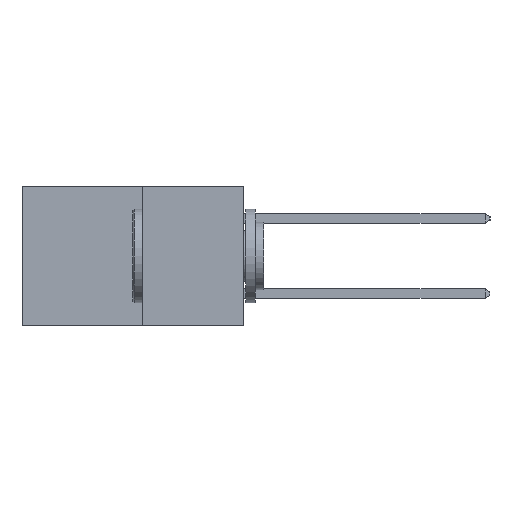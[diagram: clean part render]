
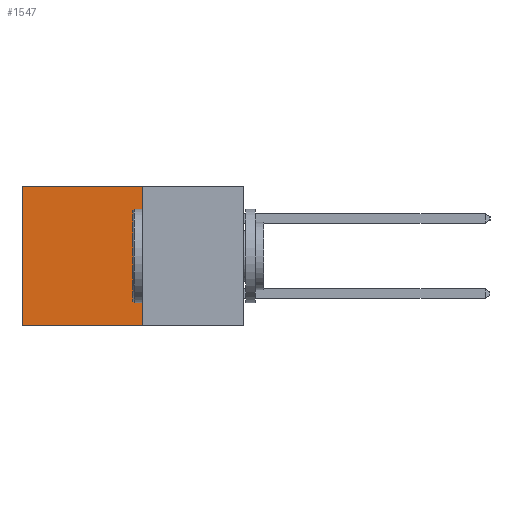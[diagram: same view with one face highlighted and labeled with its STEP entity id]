
A CAD part, left-side view. The second image highlights one B-rep face of the part: STEP entity #1547.
In plain terms, the highlighted planar face has unit normal (-1, 0, 0).
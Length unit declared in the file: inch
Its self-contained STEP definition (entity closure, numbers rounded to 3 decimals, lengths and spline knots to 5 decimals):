
#429 = DIRECTION ( 'NONE',  ( 0., 1., 0. ) ) ;
#512 = LINE ( 'NONE', #8108, #9013 ) ;
#549 = CARTESIAN_POINT ( 'NONE',  ( 0.277, 0.27, -0.37 ) ) ;
#713 = ORIENTED_EDGE ( 'NONE', *, *, #4746, .F. ) ;
#1438 = EDGE_LOOP ( 'NONE', ( #6403, #713, #5335, #3864 ) ) ;
#1547 = ADVANCED_FACE ( 'NONE', ( #10378 ), #9624, .F. ) ;
#2366 = VERTEX_POINT ( 'NONE', #4047 ) ;
#3277 = CARTESIAN_POINT ( 'NONE',  ( 0.277, 0.27, -0.37 ) ) ;
#3645 = VECTOR ( 'NONE', #9243, 39.37008 ) ;
#3669 = EDGE_CURVE ( 'NONE', #6600, #9854, #10210, .T. ) ;
#3829 = DIRECTION ( 'NONE',  ( 0., 0., -1. ) ) ;
#3864 = ORIENTED_EDGE ( 'NONE', *, *, #3669, .T. ) ;
#3939 = CARTESIAN_POINT ( 'NONE',  ( 0.277, 0.59, -0.37 ) ) ;
#4047 = CARTESIAN_POINT ( 'NONE',  ( 0.277, 0.59, -0.37 ) ) ;
#4356 = EDGE_CURVE ( 'NONE', #9854, #2366, #10320, .T. ) ;
#4531 = VECTOR ( 'NONE', #429, 39.37008 ) ;
#4746 = EDGE_CURVE ( 'NONE', #5985, #2366, #8927, .T. ) ;
#5112 = CARTESIAN_POINT ( 'NONE',  ( 0.277, 0.59, 0. ) ) ;
#5335 = ORIENTED_EDGE ( 'NONE', *, *, #10617, .F. ) ;
#5985 = VERTEX_POINT ( 'NONE', #7421 ) ;
#6403 = ORIENTED_EDGE ( 'NONE', *, *, #4356, .T. ) ;
#6469 = DIRECTION ( 'NONE',  ( 0., 0., -1. ) ) ;
#6600 = VERTEX_POINT ( 'NONE', #9084 ) ;
#6880 = DIRECTION ( 'NONE',  ( 1., 0., 0. ) ) ;
#7421 = CARTESIAN_POINT ( 'NONE',  ( 0.277, 0.27, -0.37 ) ) ;
#8101 = AXIS2_PLACEMENT_3D ( 'NONE', #3277, #6880, #6469 ) ;
#8108 = CARTESIAN_POINT ( 'NONE',  ( 0.277, 0.27, -0.37 ) ) ;
#8194 = VECTOR ( 'NONE', #3829, 39.37008 ) ;
#8927 = LINE ( 'NONE', #549, #4531 ) ;
#9013 = VECTOR ( 'NONE', #10509, 39.37008 ) ;
#9084 = CARTESIAN_POINT ( 'NONE',  ( 0.277, 0.27, 0. ) ) ;
#9150 = CARTESIAN_POINT ( 'NONE',  ( 0.277, 0.27, 0. ) ) ;
#9243 = DIRECTION ( 'NONE',  ( 0., 1., 0. ) ) ;
#9624 = PLANE ( 'NONE',  #8101 ) ;
#9854 = VERTEX_POINT ( 'NONE', #5112 ) ;
#10210 = LINE ( 'NONE', #9150, #3645 ) ;
#10320 = LINE ( 'NONE', #3939, #8194 ) ;
#10378 = FACE_OUTER_BOUND ( 'NONE', #1438, .T. ) ;
#10509 = DIRECTION ( 'NONE',  ( 0., 0., -1. ) ) ;
#10617 = EDGE_CURVE ( 'NONE', #6600, #5985, #512, .T. ) ;
